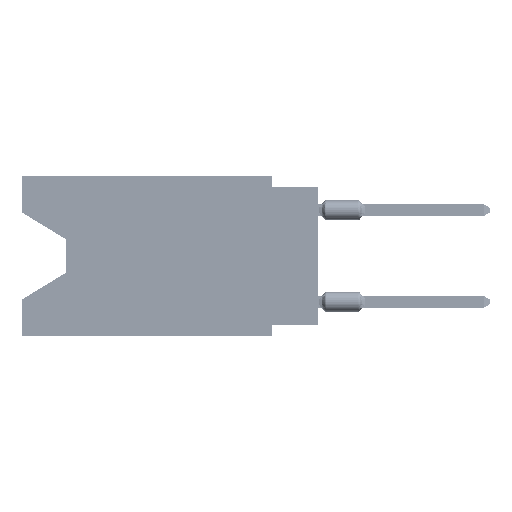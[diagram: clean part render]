
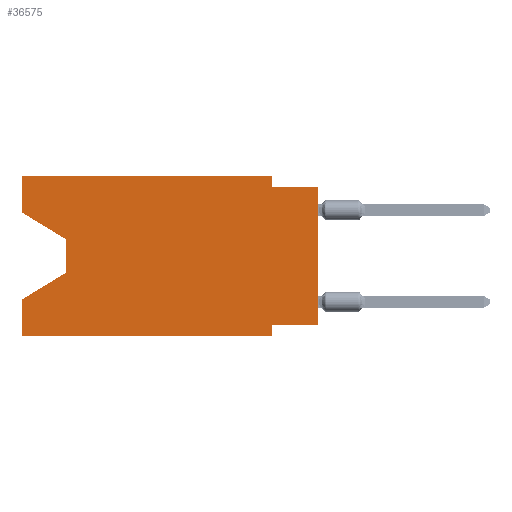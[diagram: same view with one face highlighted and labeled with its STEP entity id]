
A CAD part, left-side view. The second image highlights one B-rep face of the part: STEP entity #36575.
In plain terms, the highlighted planar face has unit normal (-1, 0, 0).
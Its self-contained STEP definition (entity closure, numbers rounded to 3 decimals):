
#650 = LINE ( 'NONE', #59775, #36142 ) ;
#1138 = CARTESIAN_POINT ( 'NONE',  ( 0., 16.383, -2.038 ) ) ;
#2521 = LINE ( 'NONE', #45207, #56553 ) ;
#2601 = VERTEX_POINT ( 'NONE', #15126 ) ;
#2786 = VECTOR ( 'NONE', #30891, 1000. ) ;
#2815 = VERTEX_POINT ( 'NONE', #3076 ) ;
#3076 = CARTESIAN_POINT ( 'NONE',  ( 0., 13.97, -5.385 ) ) ;
#3681 = EDGE_CURVE ( 'NONE', #14527, #48888, #61332, .T. ) ;
#5985 = EDGE_LOOP ( 'NONE', ( #24953, #22001, #13225, #34802, #22022, #49290, #21589, #49564, #54295, #25885, #66250, #61209 ) ) ;
#6230 = VECTOR ( 'NONE', #67680, 1000. ) ;
#6743 = CARTESIAN_POINT ( 'NONE',  ( 0., 2.54, -0.635 ) ) ;
#7470 = EDGE_CURVE ( 'NONE', #58957, #35439, #29152, .T. ) ;
#8110 = DIRECTION ( 'NONE',  ( 0., 0., -1. ) ) ;
#8825 = EDGE_CURVE ( 'NONE', #2601, #48888, #63466, .T. ) ;
#9349 = CARTESIAN_POINT ( 'NONE',  ( 0., 13.97, -3.505 ) ) ;
#9561 = DIRECTION ( 'NONE',  ( 0., 0., 1. ) ) ;
#10939 = LINE ( 'NONE', #32299, #36164 ) ;
#13225 = ORIENTED_EDGE ( 'NONE', *, *, #16721, .T. ) ;
#14008 = VERTEX_POINT ( 'NONE', #58303 ) ;
#14527 = VERTEX_POINT ( 'NONE', #6743 ) ;
#15126 = CARTESIAN_POINT ( 'NONE',  ( 0., 0., -8.255 ) ) ;
#15402 = EDGE_CURVE ( 'NONE', #50821, #45846, #650, .T. ) ;
#15684 = CARTESIAN_POINT ( 'NONE',  ( 0., 13.97, -5.385 ) ) ;
#15799 = CARTESIAN_POINT ( 'NONE',  ( 0., 13.97, -3.505 ) ) ;
#15852 = DIRECTION ( 'NONE',  ( 1., 0., 0. ) ) ;
#16721 = EDGE_CURVE ( 'NONE', #2815, #14008, #47877, .T. ) ;
#16742 = CARTESIAN_POINT ( 'NONE',  ( 0., 16.383, 0. ) ) ;
#16885 = FACE_OUTER_BOUND ( 'NONE', #5985, .T. ) ;
#18199 = VECTOR ( 'NONE', #36665, 1000. ) ;
#18315 = DIRECTION ( 'NONE',  ( 0., -1., 0. ) ) ;
#18346 = CARTESIAN_POINT ( 'NONE',  ( 0., 16.383, -2.038 ) ) ;
#19350 = VERTEX_POINT ( 'NONE', #15799 ) ;
#20315 = EDGE_CURVE ( 'NONE', #45490, #35439, #2521, .T. ) ;
#21223 = LINE ( 'NONE', #56934, #64861 ) ;
#21589 = ORIENTED_EDGE ( 'NONE', *, *, #49829, .F. ) ;
#21666 = DIRECTION ( 'NONE',  ( 0., -1., 0. ) ) ;
#22001 = ORIENTED_EDGE ( 'NONE', *, *, #22618, .T. ) ;
#22022 = ORIENTED_EDGE ( 'NONE', *, *, #7470, .T. ) ;
#22618 = EDGE_CURVE ( 'NONE', #19350, #2815, #68836, .T. ) ;
#22760 = CARTESIAN_POINT ( 'NONE',  ( 0., 2.54, -8.89 ) ) ;
#23734 = VERTEX_POINT ( 'NONE', #18346 ) ;
#24953 = ORIENTED_EDGE ( 'NONE', *, *, #59707, .T. ) ;
#25442 = DIRECTION ( 'NONE',  ( 0., 0., -1. ) ) ;
#25885 = ORIENTED_EDGE ( 'NONE', *, *, #68878, .F. ) ;
#26165 = DIRECTION ( 'NONE',  ( 0., 0., -1. ) ) ;
#29152 = LINE ( 'NONE', #50501, #2786 ) ;
#30891 = DIRECTION ( 'NONE',  ( 0., -1., 0. ) ) ;
#31417 = CARTESIAN_POINT ( 'NONE',  ( 0., 2.54, 0. ) ) ;
#32299 = CARTESIAN_POINT ( 'NONE',  ( 0., 16.383, 0. ) ) ;
#32970 = CARTESIAN_POINT ( 'NONE',  ( 0., 16.383, 0. ) ) ;
#34802 = ORIENTED_EDGE ( 'NONE', *, *, #42425, .F. ) ;
#35439 = VERTEX_POINT ( 'NONE', #22760 ) ;
#36142 = VECTOR ( 'NONE', #21666, 1000. ) ;
#36164 = VECTOR ( 'NONE', #9561, 1000. ) ;
#36575 = ADVANCED_FACE ( 'NONE', ( #16885 ), #38211, .F. ) ;
#36647 = LINE ( 'NONE', #31417, #43200 ) ;
#36665 = DIRECTION ( 'NONE',  ( 0., 0.855, -0.519 ) ) ;
#36856 = CARTESIAN_POINT ( 'NONE',  ( 0., 0., 0. ) ) ;
#38211 = PLANE ( 'NONE',  #59219 ) ;
#40791 = VECTOR ( 'NONE', #49084, 1000. ) ;
#42220 = DIRECTION ( 'NONE',  ( 0., 1., 0. ) ) ;
#42425 = EDGE_CURVE ( 'NONE', #58957, #14008, #10939, .T. ) ;
#42646 = DIRECTION ( 'NONE',  ( 0., 0., 1. ) ) ;
#43200 = VECTOR ( 'NONE', #26165, 1000. ) ;
#45207 = CARTESIAN_POINT ( 'NONE',  ( 0., 2.54, -8.89 ) ) ;
#45490 = VERTEX_POINT ( 'NONE', #62497 ) ;
#45554 = CARTESIAN_POINT ( 'NONE',  ( 0., 0., -0.635 ) ) ;
#45846 = VERTEX_POINT ( 'NONE', #62421 ) ;
#46873 = EDGE_CURVE ( 'NONE', #23734, #50821, #48595, .T. ) ;
#47354 = DIRECTION ( 'NONE',  ( 0., 0., -1. ) ) ;
#47877 = LINE ( 'NONE', #15684, #18199 ) ;
#48595 = LINE ( 'NONE', #16742, #54624 ) ;
#48888 = VERTEX_POINT ( 'NONE', #45554 ) ;
#49084 = DIRECTION ( 'NONE',  ( 0., -0.855, -0.519 ) ) ;
#49289 = CARTESIAN_POINT ( 'NONE',  ( 0., 16.383, 0. ) ) ;
#49290 = ORIENTED_EDGE ( 'NONE', *, *, #20315, .F. ) ;
#49564 = ORIENTED_EDGE ( 'NONE', *, *, #8825, .T. ) ;
#49829 = EDGE_CURVE ( 'NONE', #2601, #45490, #21223, .T. ) ;
#50501 = CARTESIAN_POINT ( 'NONE',  ( 0., 16.383, -8.89 ) ) ;
#50821 = VERTEX_POINT ( 'NONE', #49289 ) ;
#54295 = ORIENTED_EDGE ( 'NONE', *, *, #3681, .F. ) ;
#54624 = VECTOR ( 'NONE', #42646, 1000. ) ;
#56553 = VECTOR ( 'NONE', #8110, 1000. ) ;
#56934 = CARTESIAN_POINT ( 'NONE',  ( 0., 0., -8.255 ) ) ;
#58303 = CARTESIAN_POINT ( 'NONE',  ( 0., 16.383, -6.852 ) ) ;
#58957 = VERTEX_POINT ( 'NONE', #66375 ) ;
#59219 = AXIS2_PLACEMENT_3D ( 'NONE', #32970, #15852, #47354 ) ;
#59243 = LINE ( 'NONE', #1138, #40791 ) ;
#59316 = VECTOR ( 'NONE', #18315, 1000. ) ;
#59707 = EDGE_CURVE ( 'NONE', #23734, #19350, #59243, .T. ) ;
#59775 = CARTESIAN_POINT ( 'NONE',  ( 0., 16.383, 0. ) ) ;
#59945 = VECTOR ( 'NONE', #25442, 1000. ) ;
#61209 = ORIENTED_EDGE ( 'NONE', *, *, #46873, .F. ) ;
#61332 = LINE ( 'NONE', #66260, #59316 ) ;
#62421 = CARTESIAN_POINT ( 'NONE',  ( 0., 2.54, 0. ) ) ;
#62497 = CARTESIAN_POINT ( 'NONE',  ( 0., 2.54, -8.255 ) ) ;
#63466 = LINE ( 'NONE', #36856, #6230 ) ;
#64861 = VECTOR ( 'NONE', #42220, 1000. ) ;
#66250 = ORIENTED_EDGE ( 'NONE', *, *, #15402, .F. ) ;
#66260 = CARTESIAN_POINT ( 'NONE',  ( 0., 0., -0.635 ) ) ;
#66375 = CARTESIAN_POINT ( 'NONE',  ( 0., 16.383, -8.89 ) ) ;
#67680 = DIRECTION ( 'NONE',  ( 0., 0., 1. ) ) ;
#68836 = LINE ( 'NONE', #9349, #59945 ) ;
#68878 = EDGE_CURVE ( 'NONE', #45846, #14527, #36647, .T. ) ;
